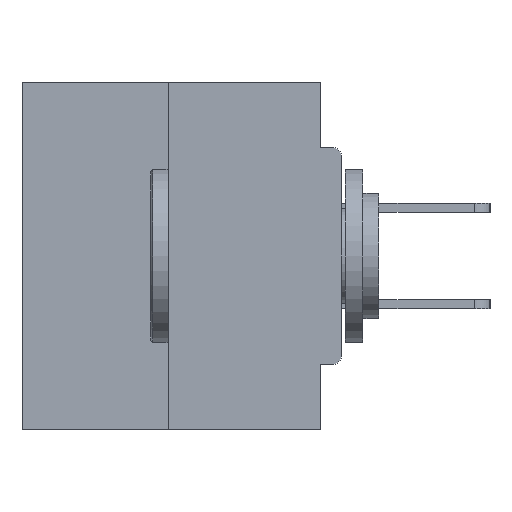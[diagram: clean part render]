
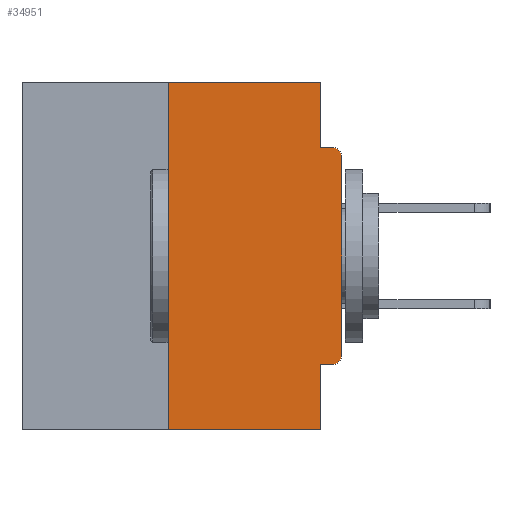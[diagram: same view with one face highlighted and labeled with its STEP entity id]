
A CAD part, left-side view. The second image highlights one B-rep face of the part: STEP entity #34951.
In plain terms, the highlighted planar face has unit normal (-1, 0, 0).
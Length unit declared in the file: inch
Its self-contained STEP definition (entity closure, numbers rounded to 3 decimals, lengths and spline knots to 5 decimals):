
#70 = CIRCLE ( 'NONE', #20139, 0.015 ) ;
#107 = CARTESIAN_POINT ( 'NONE',  ( 0., 0.46, -0.5 ) ) ;
#777 = EDGE_CURVE ( 'NONE', #5210, #16099, #14019, .T. ) ;
#830 = DIRECTION ( 'NONE',  ( 1., 0., 0. ) ) ;
#952 = CARTESIAN_POINT ( 'NONE',  ( 0., 0., -0.0935 ) ) ;
#1013 = AXIS2_PLACEMENT_3D ( 'NONE', #31277, #20456, #45661 ) ;
#1127 = VERTEX_POINT ( 'NONE', #9267 ) ;
#1403 = VECTOR ( 'NONE', #24186, 39.37008 ) ;
#2461 = DIRECTION ( 'NONE',  ( 0., 0., -1. ) ) ;
#3369 = VERTEX_POINT ( 'NONE', #42751 ) ;
#3539 = DIRECTION ( 'NONE',  ( 0., 0., 1. ) ) ;
#4442 = ORIENTED_EDGE ( 'NONE', *, *, #17109, .T. ) ;
#5210 = VERTEX_POINT ( 'NONE', #44894 ) ;
#5970 = DIRECTION ( 'NONE',  ( 0., 0., 1. ) ) ;
#6184 = CARTESIAN_POINT ( 'NONE',  ( 0., 0.015, -0.4065 ) ) ;
#6200 = LINE ( 'NONE', #107, #7327 ) ;
#7327 = VECTOR ( 'NONE', #17659, 39.37008 ) ;
#8107 = CARTESIAN_POINT ( 'NONE',  ( 0., 0.031, 0. ) ) ;
#8483 = CARTESIAN_POINT ( 'NONE',  ( 0., 0., -0.3915 ) ) ;
#8520 = CARTESIAN_POINT ( 'NONE',  ( 0., 0.031, 0. ) ) ;
#9267 = CARTESIAN_POINT ( 'NONE',  ( 0., 0.031, -0.4065 ) ) ;
#11013 = CARTESIAN_POINT ( 'NONE',  ( 0., 0.46, 0. ) ) ;
#12230 = LINE ( 'NONE', #30965, #34198 ) ;
#12687 = ORIENTED_EDGE ( 'NONE', *, *, #38464, .F. ) ;
#14019 = LINE ( 'NONE', #25028, #28064 ) ;
#14716 = CIRCLE ( 'NONE', #1013, 0.015 ) ;
#14834 = LINE ( 'NONE', #38502, #1403 ) ;
#15003 = LINE ( 'NONE', #17879, #44698 ) ;
#15321 = LINE ( 'NONE', #952, #33787 ) ;
#15515 = DIRECTION ( 'NONE',  ( 0., -1., 0. ) ) ;
#16099 = VERTEX_POINT ( 'NONE', #18045 ) ;
#17109 = EDGE_CURVE ( 'NONE', #31421, #28304, #14716, .T. ) ;
#17659 = DIRECTION ( 'NONE',  ( 0., -1., 0. ) ) ;
#17879 = CARTESIAN_POINT ( 'NONE',  ( 0., 0., -0.4065 ) ) ;
#18045 = CARTESIAN_POINT ( 'NONE',  ( 0., 0.25, 0. ) ) ;
#18066 = ORIENTED_EDGE ( 'NONE', *, *, #25817, .T. ) ;
#18443 = LINE ( 'NONE', #20231, #24638 ) ;
#19814 = VERTEX_POINT ( 'NONE', #33395 ) ;
#20139 = AXIS2_PLACEMENT_3D ( 'NONE', #35245, #38806, #27756 ) ;
#20231 = CARTESIAN_POINT ( 'NONE',  ( 0., 0., 0. ) ) ;
#20255 = ORIENTED_EDGE ( 'NONE', *, *, #34416, .T. ) ;
#20456 = DIRECTION ( 'NONE',  ( -1., 0., 0. ) ) ;
#21711 = DIRECTION ( 'NONE',  ( 0., 0., -1. ) ) ;
#22878 = AXIS2_PLACEMENT_3D ( 'NONE', #11013, #830, #21711 ) ;
#23915 = LINE ( 'NONE', #8520, #44617 ) ;
#23994 = EDGE_CURVE ( 'NONE', #16099, #30664, #14834, .T. ) ;
#24186 = DIRECTION ( 'NONE',  ( 0., -1., 0. ) ) ;
#24638 = VECTOR ( 'NONE', #5970, 39.37008 ) ;
#25028 = CARTESIAN_POINT ( 'NONE',  ( 0., 0.25, 0. ) ) ;
#25621 = PLANE ( 'NONE',  #22878 ) ;
#25817 = EDGE_CURVE ( 'NONE', #34466, #26887, #70, .T. ) ;
#26263 = ORIENTED_EDGE ( 'NONE', *, *, #26572, .F. ) ;
#26572 = EDGE_CURVE ( 'NONE', #1127, #3369, #12230, .T. ) ;
#26887 = VERTEX_POINT ( 'NONE', #28716 ) ;
#27756 = DIRECTION ( 'NONE',  ( 0., 0., -1. ) ) ;
#28064 = VECTOR ( 'NONE', #3539, 39.37008 ) ;
#28304 = VERTEX_POINT ( 'NONE', #8483 ) ;
#28716 = CARTESIAN_POINT ( 'NONE',  ( 0., 0.015, -0.0935 ) ) ;
#30054 = EDGE_CURVE ( 'NONE', #30664, #19814, #23915, .T. ) ;
#30108 = EDGE_LOOP ( 'NONE', ( #45347, #33346, #40913, #26263, #35146, #4442, #20255, #18066, #12687, #35192 ) ) ;
#30664 = VERTEX_POINT ( 'NONE', #8107 ) ;
#30965 = CARTESIAN_POINT ( 'NONE',  ( 0., 0.031, -0.5 ) ) ;
#31277 = CARTESIAN_POINT ( 'NONE',  ( 0., 0.015, -0.3915 ) ) ;
#31421 = VERTEX_POINT ( 'NONE', #6184 ) ;
#32301 = DIRECTION ( 'NONE',  ( 0., 1., 0. ) ) ;
#33346 = ORIENTED_EDGE ( 'NONE', *, *, #777, .F. ) ;
#33395 = CARTESIAN_POINT ( 'NONE',  ( 0., 0.031, -0.0935 ) ) ;
#33556 = FACE_OUTER_BOUND ( 'NONE', #30108, .T. ) ;
#33787 = VECTOR ( 'NONE', #15515, 39.37008 ) ;
#34198 = VECTOR ( 'NONE', #2461, 39.37008 ) ;
#34416 = EDGE_CURVE ( 'NONE', #28304, #34466, #18443, .T. ) ;
#34466 = VERTEX_POINT ( 'NONE', #42431 ) ;
#34951 = ADVANCED_FACE ( 'NONE', ( #33556 ), #25621, .F. ) ;
#35146 = ORIENTED_EDGE ( 'NONE', *, *, #44646, .F. ) ;
#35192 = ORIENTED_EDGE ( 'NONE', *, *, #30054, .F. ) ;
#35245 = CARTESIAN_POINT ( 'NONE',  ( 0., 0.015, -0.1085 ) ) ;
#37661 = DIRECTION ( 'NONE',  ( 0., 0., -1. ) ) ;
#38464 = EDGE_CURVE ( 'NONE', #19814, #26887, #15321, .T. ) ;
#38502 = CARTESIAN_POINT ( 'NONE',  ( 0., 0.46, 0. ) ) ;
#38806 = DIRECTION ( 'NONE',  ( -1., 0., 0. ) ) ;
#40913 = ORIENTED_EDGE ( 'NONE', *, *, #41901, .T. ) ;
#41901 = EDGE_CURVE ( 'NONE', #5210, #3369, #6200, .T. ) ;
#42431 = CARTESIAN_POINT ( 'NONE',  ( 0., 0., -0.1085 ) ) ;
#42751 = CARTESIAN_POINT ( 'NONE',  ( 0., 0.031, -0.5 ) ) ;
#44617 = VECTOR ( 'NONE', #37661, 39.37008 ) ;
#44646 = EDGE_CURVE ( 'NONE', #31421, #1127, #15003, .T. ) ;
#44698 = VECTOR ( 'NONE', #32301, 39.37008 ) ;
#44894 = CARTESIAN_POINT ( 'NONE',  ( 0., 0.25, -0.5 ) ) ;
#45347 = ORIENTED_EDGE ( 'NONE', *, *, #23994, .F. ) ;
#45661 = DIRECTION ( 'NONE',  ( 0., 0., -1. ) ) ;
